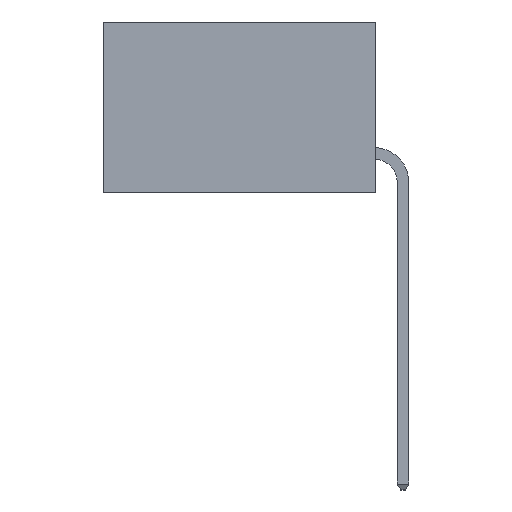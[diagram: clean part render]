
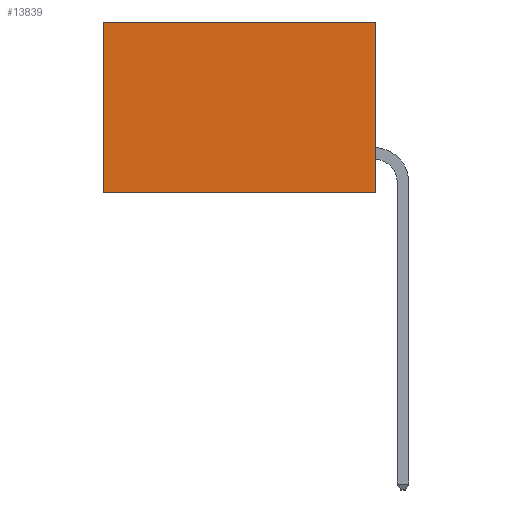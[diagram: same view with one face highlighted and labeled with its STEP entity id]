
A CAD part, left-side view. The second image highlights one B-rep face of the part: STEP entity #13839.
In plain terms, the highlighted planar face has unit normal (-1, 0, 0).
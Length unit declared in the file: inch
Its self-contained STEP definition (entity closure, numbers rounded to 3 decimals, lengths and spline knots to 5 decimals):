
#44 = DIRECTION ( 'NONE',  ( 0., 0., -1. ) ) ;
#88 = EDGE_CURVE ( 'NONE', #3751, #25122, #13838, .T. ) ;
#1819 = ORIENTED_EDGE ( 'NONE', *, *, #11781, .T. ) ;
#2665 = VECTOR ( 'NONE', #22906, 39.37008 ) ;
#3751 = VERTEX_POINT ( 'NONE', #28331 ) ;
#5997 = LINE ( 'NONE', #8944, #29037 ) ;
#7013 = DIRECTION ( 'NONE',  ( 0., 1., 0. ) ) ;
#8502 = DIRECTION ( 'NONE',  ( 0., 1., 0. ) ) ;
#8591 = DIRECTION ( 'NONE',  ( 0., 0., -1. ) ) ;
#8944 = CARTESIAN_POINT ( 'NONE',  ( 0.277, 0.59, -0.37 ) ) ;
#9649 = PLANE ( 'NONE',  #24495 ) ;
#10510 = EDGE_CURVE ( 'NONE', #20392, #19321, #5997, .T. ) ;
#10609 = ORIENTED_EDGE ( 'NONE', *, *, #88, .F. ) ;
#10736 = ORIENTED_EDGE ( 'NONE', *, *, #25960, .F. ) ;
#11781 = EDGE_CURVE ( 'NONE', #3751, #20392, #21901, .T. ) ;
#12066 = CARTESIAN_POINT ( 'NONE',  ( 0.277, 0., -0.37 ) ) ;
#13838 = LINE ( 'NONE', #28520, #2665 ) ;
#13839 = ADVANCED_FACE ( 'NONE', ( #25961 ), #9649, .F. ) ;
#14395 = DIRECTION ( 'NONE',  ( 1., 0., 0. ) ) ;
#15777 = VECTOR ( 'NONE', #7013, 39.37008 ) ;
#17927 = LINE ( 'NONE', #22378, #24714 ) ;
#19321 = VERTEX_POINT ( 'NONE', #23538 ) ;
#19734 = CARTESIAN_POINT ( 'NONE',  ( 0.277, 0., -0.37 ) ) ;
#20392 = VERTEX_POINT ( 'NONE', #22916 ) ;
#21901 = LINE ( 'NONE', #23138, #15777 ) ;
#22378 = CARTESIAN_POINT ( 'NONE',  ( 0.277, 0., -0.37 ) ) ;
#22906 = DIRECTION ( 'NONE',  ( 0., 0., -1. ) ) ;
#22916 = CARTESIAN_POINT ( 'NONE',  ( 0.277, 0.59, 0. ) ) ;
#23079 = ORIENTED_EDGE ( 'NONE', *, *, #10510, .T. ) ;
#23138 = CARTESIAN_POINT ( 'NONE',  ( 0.277, 0., 0. ) ) ;
#23538 = CARTESIAN_POINT ( 'NONE',  ( 0.277, 0.59, -0.37 ) ) ;
#24495 = AXIS2_PLACEMENT_3D ( 'NONE', #12066, #14395, #44 ) ;
#24714 = VECTOR ( 'NONE', #8502, 39.37008 ) ;
#25122 = VERTEX_POINT ( 'NONE', #19734 ) ;
#25960 = EDGE_CURVE ( 'NONE', #25122, #19321, #17927, .T. ) ;
#25961 = FACE_OUTER_BOUND ( 'NONE', #28902, .T. ) ;
#28331 = CARTESIAN_POINT ( 'NONE',  ( 0.277, 0., 0. ) ) ;
#28520 = CARTESIAN_POINT ( 'NONE',  ( 0.277, 0., -0.37 ) ) ;
#28902 = EDGE_LOOP ( 'NONE', ( #23079, #10736, #10609, #1819 ) ) ;
#29037 = VECTOR ( 'NONE', #8591, 39.37008 ) ;
